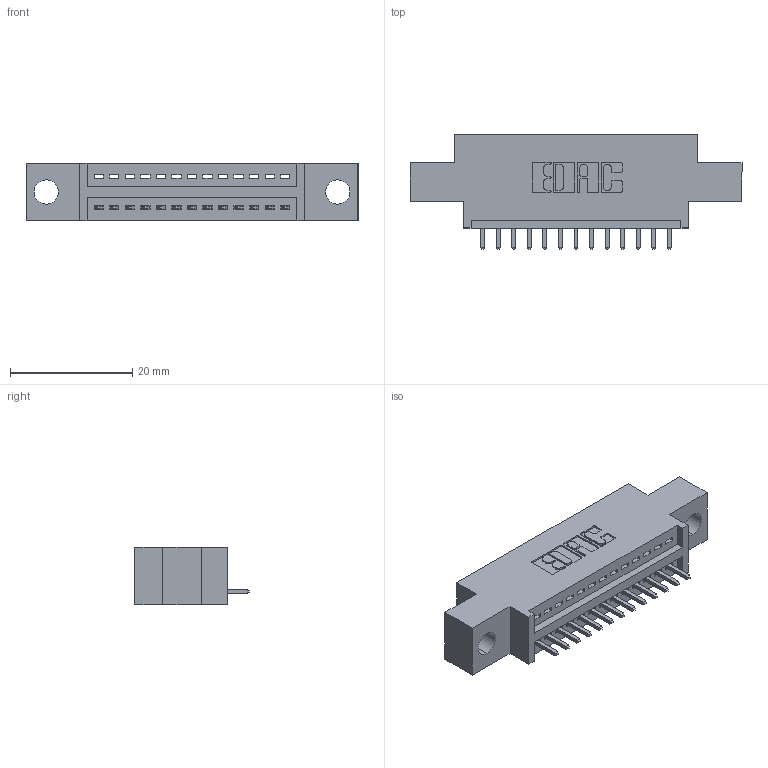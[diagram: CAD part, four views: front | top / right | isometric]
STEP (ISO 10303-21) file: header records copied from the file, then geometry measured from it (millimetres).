
FILE_DESCRIPTION (( 'STEP AP203' ), '1' );
FILE_NAME ('395-013-521-604.STEP', '2021-05-31T14:18:46', ( '' ), ( '' ), 'SwSTEP 2.0', 'SolidWorks 2020', '' );
FILE_SCHEMA (( 'CONFIG_CONTROL_DESIGN' ));
Length unit declared in the file: inch
Products named in the file (3): 395-013-521-604; 345 Part_0.170 Offset - 0.156 Dia-TI; 345-292-001_345-293-121
Assembly tree (14 placements, depth 2):
  395-013-521-604
    345 Part_0.170 Offset - 0.156 Dia-TI
    345-292-001_345-293-121  x13
Bounding box: 54.23 x 18.72 x 9.4 mm (x, y, z)
Volume: 4656.8 mm3; surface area: 5618.8 mm2
Topology: 14 solids, 14 shells, 898 faces, 2677 edges, 1766 vertices
Faces by surface type: plane 618, cylinder 280
Entity records: 14257 total; most frequent: CARTESIAN_POINT 2481, ORIENTED_EDGE 2426, DIRECTION 2207, EDGE_CURVE 1213, VECTOR 1029, LINE 1029, VERTEX_POINT 806, AXIS2_PLACEMENT_3D 589
